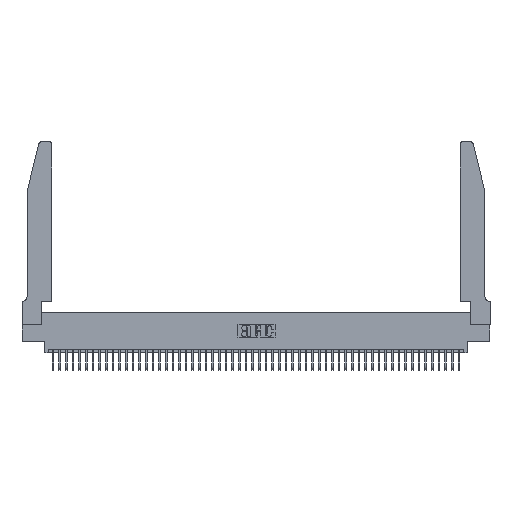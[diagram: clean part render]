
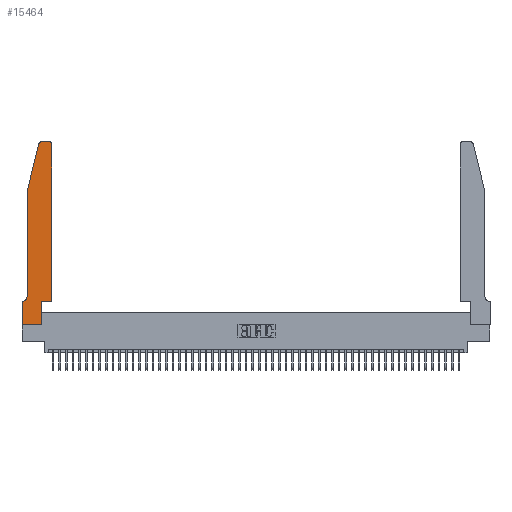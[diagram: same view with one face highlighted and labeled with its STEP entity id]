
A CAD part, top view. The second image highlights one B-rep face of the part: STEP entity #15464.
In plain terms, the highlighted planar face has unit normal (0, 0, 1).
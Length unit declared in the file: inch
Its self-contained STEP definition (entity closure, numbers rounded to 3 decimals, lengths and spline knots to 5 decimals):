
#66 = VECTOR ( 'NONE', #39029, 39.37008 ) ;
#123 = ORIENTED_EDGE ( 'NONE', *, *, #25489, .T. ) ;
#179 = CARTESIAN_POINT ( 'NONE',  ( 0.4505, 2.72, 0.37 ) ) ;
#224 = CARTESIAN_POINT ( 'NONE',  ( 0.2865, 0.35, 0.37 ) ) ;
#1008 = CARTESIAN_POINT ( 'NONE',  ( 0.0055, 0.35, 0.37 ) ) ;
#1361 = EDGE_CURVE ( 'NONE', #42878, #17170, #47440, .T. ) ;
#2831 = CARTESIAN_POINT ( 'NONE',  ( 0.4505, 0.35, 0.37 ) ) ;
#3920 = CARTESIAN_POINT ( 'NONE',  ( 0.25487, 2.72718, 0.37 ) ) ;
#4098 = VECTOR ( 'NONE', #37188, 39.37008 ) ;
#4320 = VERTEX_POINT ( 'NONE', #24399 ) ;
#5133 = VERTEX_POINT ( 'NONE', #1008 ) ;
#7559 = EDGE_CURVE ( 'NONE', #35892, #27208, #17896, .T. ) ;
#8111 = DIRECTION ( 'NONE',  ( 1., 0., 0. ) ) ;
#8317 = VECTOR ( 'NONE', #21419, 39.37008 ) ;
#9812 = ORIENTED_EDGE ( 'NONE', *, *, #7559, .T. ) ;
#10046 = DIRECTION ( 'NONE',  ( 0., 1., 0. ) ) ;
#10865 = AXIS2_PLACEMENT_3D ( 'NONE', #38484, #14054, #14229 ) ;
#11355 = CARTESIAN_POINT ( 'NONE',  ( 0., 0., 0.37 ) ) ;
#11518 = CARTESIAN_POINT ( 'NONE',  ( 0.4505, 0.35, 0.37 ) ) ;
#11794 = ORIENTED_EDGE ( 'NONE', *, *, #35201, .T. ) ;
#12619 = CIRCLE ( 'NONE', #43184, 0.03 ) ;
#12776 = LINE ( 'NONE', #22714, #66 ) ;
#13244 = ORIENTED_EDGE ( 'NONE', *, *, #15275, .T. ) ;
#13393 = DIRECTION ( 'NONE',  ( -1., 0., 0. ) ) ;
#13657 = CIRCLE ( 'NONE', #46515, 0.03 ) ;
#14054 = DIRECTION ( 'NONE',  ( 0., 0., -1. ) ) ;
#14229 = DIRECTION ( 'NONE',  ( -1., 0., 0. ) ) ;
#14385 = EDGE_CURVE ( 'NONE', #24662, #18924, #41668, .T. ) ;
#14583 = DIRECTION ( 'NONE',  ( -1., 0., 0. ) ) ;
#14952 = LINE ( 'NONE', #49392, #44759 ) ;
#15275 = EDGE_CURVE ( 'NONE', #27208, #5133, #23709, .T. ) ;
#15464 = ADVANCED_FACE ( 'NONE', ( #44052 ), #16290, .T. ) ;
#15759 = DIRECTION ( 'NONE',  ( 1., 0., 0. ) ) ;
#16290 = PLANE ( 'NONE',  #31612 ) ;
#16648 = DIRECTION ( 'NONE',  ( 0., 0., 1. ) ) ;
#17170 = VERTEX_POINT ( 'NONE', #11355 ) ;
#17726 = VECTOR ( 'NONE', #34730, 39.37008 ) ;
#17896 = LINE ( 'NONE', #25272, #8317 ) ;
#18716 = CARTESIAN_POINT ( 'NONE',  ( 0.0755, 2., 0.37 ) ) ;
#18924 = VERTEX_POINT ( 'NONE', #224 ) ;
#20001 = VERTEX_POINT ( 'NONE', #179 ) ;
#20660 = VERTEX_POINT ( 'NONE', #33081 ) ;
#20813 = VECTOR ( 'NONE', #28012, 39.37008 ) ;
#21419 = DIRECTION ( 'NONE',  ( 0., -1., 0. ) ) ;
#22714 = CARTESIAN_POINT ( 'NONE',  ( 0., 0., 0.37 ) ) ;
#23166 = ORIENTED_EDGE ( 'NONE', *, *, #27943, .T. ) ;
#23374 = EDGE_CURVE ( 'NONE', #18924, #32697, #31571, .T. ) ;
#23709 = CIRCLE ( 'NONE', #10865, 0.07 ) ;
#24241 = ORIENTED_EDGE ( 'NONE', *, *, #37805, .T. ) ;
#24253 = CARTESIAN_POINT ( 'NONE',  ( 0.4205, 2.72, 0.37 ) ) ;
#24399 = CARTESIAN_POINT ( 'NONE',  ( 0.4205, 2.75, 0.37 ) ) ;
#24662 = VERTEX_POINT ( 'NONE', #37317 ) ;
#24718 = DIRECTION ( 'NONE',  ( 0., -1., 0. ) ) ;
#25272 = CARTESIAN_POINT ( 'NONE',  ( 0.0755, 2., 0.37 ) ) ;
#25489 = EDGE_CURVE ( 'NONE', #5133, #42878, #47782, .T. ) ;
#26117 = EDGE_LOOP ( 'NONE', ( #32797, #49496, #11794, #9812, #13244, #123, #48054, #37757, #43458, #34785, #23166, #24241 ) ) ;
#26128 = CARTESIAN_POINT ( 'NONE',  ( 0.4505, 0.35, 0.37 ) ) ;
#27208 = VERTEX_POINT ( 'NONE', #38894 ) ;
#27943 = EDGE_CURVE ( 'NONE', #32697, #20001, #39341, .T. ) ;
#28012 = DIRECTION ( 'NONE',  ( 1., 0., 0. ) ) ;
#28472 = CARTESIAN_POINT ( 'NONE',  ( 0., 0.35, 0.37 ) ) ;
#29689 = CARTESIAN_POINT ( 'NONE',  ( 0.284, 2.72, 0.37 ) ) ;
#30203 = EDGE_CURVE ( 'NONE', #4320, #20660, #14952, .T. ) ;
#31571 = LINE ( 'NONE', #11518, #20813 ) ;
#31612 = AXIS2_PLACEMENT_3D ( 'NONE', #28472, #40604, #15759 ) ;
#32697 = VERTEX_POINT ( 'NONE', #26128 ) ;
#32797 = ORIENTED_EDGE ( 'NONE', *, *, #30203, .T. ) ;
#33081 = CARTESIAN_POINT ( 'NONE',  ( 0.284, 2.75, 0.37 ) ) ;
#33464 = DIRECTION ( 'NONE',  ( 1., 0., 0. ) ) ;
#34730 = DIRECTION ( 'NONE',  ( 0., 1., 0. ) ) ;
#34785 = ORIENTED_EDGE ( 'NONE', *, *, #23374, .T. ) ;
#35201 = EDGE_CURVE ( 'NONE', #36307, #35892, #46646, .T. ) ;
#35204 = EDGE_CURVE ( 'NONE', #20660, #36307, #13657, .T. ) ;
#35690 = VECTOR ( 'NONE', #14583, 39.37008 ) ;
#35892 = VERTEX_POINT ( 'NONE', #18716 ) ;
#36307 = VERTEX_POINT ( 'NONE', #3920 ) ;
#37188 = DIRECTION ( 'NONE',  ( -0.239, -0.971, 0. ) ) ;
#37317 = CARTESIAN_POINT ( 'NONE',  ( 0.2865, 0., 0.37 ) ) ;
#37757 = ORIENTED_EDGE ( 'NONE', *, *, #51910, .T. ) ;
#37783 = CARTESIAN_POINT ( 'NONE',  ( 0., 0.35, 0.37 ) ) ;
#37805 = EDGE_CURVE ( 'NONE', #20001, #4320, #12619, .T. ) ;
#37878 = VECTOR ( 'NONE', #24718, 39.37008 ) ;
#38484 = CARTESIAN_POINT ( 'NONE',  ( 0.0055, 0.42, 0.37 ) ) ;
#38894 = CARTESIAN_POINT ( 'NONE',  ( 0.0755, 0.42, 0.37 ) ) ;
#39029 = DIRECTION ( 'NONE',  ( 1., 0., 0. ) ) ;
#39341 = LINE ( 'NONE', #2831, #17726 ) ;
#40604 = DIRECTION ( 'NONE',  ( 0., 0., 1. ) ) ;
#41453 = CARTESIAN_POINT ( 'NONE',  ( 0., 0., 0.37 ) ) ;
#41668 = LINE ( 'NONE', #42237, #48614 ) ;
#42237 = CARTESIAN_POINT ( 'NONE',  ( 0.2865, 0.35, 0.37 ) ) ;
#42878 = VERTEX_POINT ( 'NONE', #37783 ) ;
#43167 = CARTESIAN_POINT ( 'NONE',  ( 0.0755, 0.35, 0.37 ) ) ;
#43184 = AXIS2_PLACEMENT_3D ( 'NONE', #24253, #16648, #8111 ) ;
#43458 = ORIENTED_EDGE ( 'NONE', *, *, #14385, .T. ) ;
#44052 = FACE_OUTER_BOUND ( 'NONE', #26117, .T. ) ;
#44759 = VECTOR ( 'NONE', #13393, 39.37008 ) ;
#45534 = DIRECTION ( 'NONE',  ( 0., 0., 1. ) ) ;
#46515 = AXIS2_PLACEMENT_3D ( 'NONE', #29689, #45534, #33464 ) ;
#46646 = LINE ( 'NONE', #49273, #4098 ) ;
#47440 = LINE ( 'NONE', #41453, #37878 ) ;
#47782 = LINE ( 'NONE', #43167, #35690 ) ;
#48054 = ORIENTED_EDGE ( 'NONE', *, *, #1361, .T. ) ;
#48614 = VECTOR ( 'NONE', #10046, 39.37008 ) ;
#49273 = CARTESIAN_POINT ( 'NONE',  ( 0.0755, 2., 0.37 ) ) ;
#49392 = CARTESIAN_POINT ( 'NONE',  ( 0.2605, 2.75, 0.37 ) ) ;
#49496 = ORIENTED_EDGE ( 'NONE', *, *, #35204, .T. ) ;
#51910 = EDGE_CURVE ( 'NONE', #17170, #24662, #12776, .T. ) ;
